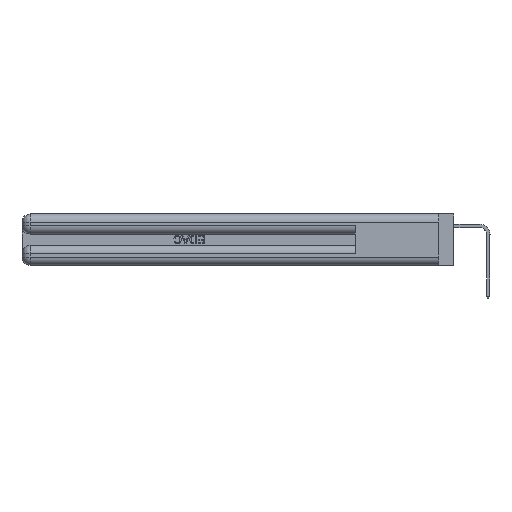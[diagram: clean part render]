
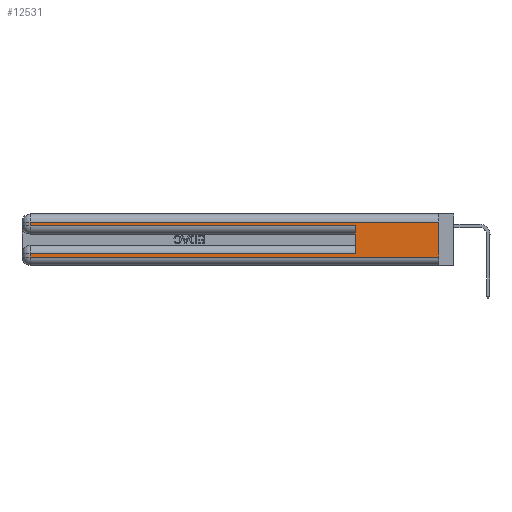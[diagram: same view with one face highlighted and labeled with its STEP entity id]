
A CAD part, left-side view. The second image highlights one B-rep face of the part: STEP entity #12531.
In plain terms, the highlighted planar face has unit normal (-1, 0, 0).
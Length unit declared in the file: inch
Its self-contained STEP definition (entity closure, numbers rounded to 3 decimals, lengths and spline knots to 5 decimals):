
#969 = CARTESIAN_POINT ( 'NONE',  ( 0., 0., 0.06 ) ) ;
#1261 = CARTESIAN_POINT ( 'NONE',  ( 0., 0., 0.37 ) ) ;
#1584 = LINE ( 'NONE', #9420, #37589 ) ;
#1821 = EDGE_CURVE ( 'NONE', #5785, #28528, #43204, .T. ) ;
#3249 = AXIS2_PLACEMENT_3D ( 'NONE', #1261, #8359, #31942 ) ;
#4107 = DIRECTION ( 'NONE',  ( 0., 1., 0. ) ) ;
#5298 = ORIENTED_EDGE ( 'NONE', *, *, #1821, .T. ) ;
#5785 = VERTEX_POINT ( 'NONE', #9802 ) ;
#6307 = VECTOR ( 'NONE', #21690, 39.37008 ) ;
#7692 = VECTOR ( 'NONE', #4107, 39.37008 ) ;
#8278 = EDGE_CURVE ( 'NONE', #22062, #12574, #39935, .T. ) ;
#8359 = DIRECTION ( 'NONE',  ( 1., 0., 0. ) ) ;
#9420 = CARTESIAN_POINT ( 'NONE',  ( 0., 2.94, 0.37 ) ) ;
#9802 = CARTESIAN_POINT ( 'NONE',  ( 0., 2.94, 0.085 ) ) ;
#10342 = CARTESIAN_POINT ( 'NONE',  ( 0., 2.94, 0.37 ) ) ;
#11108 = EDGE_CURVE ( 'NONE', #43314, #23502, #1584, .T. ) ;
#12459 = LINE ( 'NONE', #22307, #20399 ) ;
#12531 = ADVANCED_FACE ( 'NONE', ( #15473 ), #28605, .F. ) ;
#12574 = VERTEX_POINT ( 'NONE', #22025 ) ;
#12840 = DIRECTION ( 'NONE',  ( 0., 0., -1. ) ) ;
#12875 = DIRECTION ( 'NONE',  ( 0., 0., -1. ) ) ;
#13532 = DIRECTION ( 'NONE',  ( 0., -1., 0. ) ) ;
#13911 = CARTESIAN_POINT ( 'NONE',  ( 0., 0.6, 0.085 ) ) ;
#14051 = EDGE_CURVE ( 'NONE', #23502, #34182, #17973, .T. ) ;
#14349 = CARTESIAN_POINT ( 'NONE',  ( 0., 2.94, 0.06 ) ) ;
#15473 = FACE_OUTER_BOUND ( 'NONE', #43568, .T. ) ;
#15482 = CARTESIAN_POINT ( 'NONE',  ( 0., 0., 0.31 ) ) ;
#16345 = VERTEX_POINT ( 'NONE', #13911 ) ;
#16798 = LINE ( 'NONE', #21111, #7692 ) ;
#16910 = VECTOR ( 'NONE', #13532, 39.37008 ) ;
#17183 = DIRECTION ( 'NONE',  ( 0., 0., -1. ) ) ;
#17227 = ORIENTED_EDGE ( 'NONE', *, *, #32364, .T. ) ;
#17973 = LINE ( 'NONE', #20312, #16910 ) ;
#18934 = LINE ( 'NONE', #969, #37772 ) ;
#18978 = CARTESIAN_POINT ( 'NONE',  ( 0., 2.94, 0.31 ) ) ;
#19569 = EDGE_CURVE ( 'NONE', #16345, #5785, #12459, .T. ) ;
#20312 = CARTESIAN_POINT ( 'NONE',  ( 0., 0., 0.285 ) ) ;
#20399 = VECTOR ( 'NONE', #38959, 39.37008 ) ;
#21111 = CARTESIAN_POINT ( 'NONE',  ( 0., 0., 0.31 ) ) ;
#21474 = ORIENTED_EDGE ( 'NONE', *, *, #14051, .T. ) ;
#21554 = CARTESIAN_POINT ( 'NONE',  ( 0., 0.6, 0.145 ) ) ;
#21690 = DIRECTION ( 'NONE',  ( 0., 0., 1. ) ) ;
#22025 = CARTESIAN_POINT ( 'NONE',  ( 0., 0., 0.06 ) ) ;
#22062 = VERTEX_POINT ( 'NONE', #15482 ) ;
#22307 = CARTESIAN_POINT ( 'NONE',  ( 0., 0., 0.085 ) ) ;
#23502 = VERTEX_POINT ( 'NONE', #33559 ) ;
#26377 = CARTESIAN_POINT ( 'NONE',  ( 0., 0., 0.37 ) ) ;
#28528 = VERTEX_POINT ( 'NONE', #14349 ) ;
#28605 = PLANE ( 'NONE',  #3249 ) ;
#30131 = EDGE_CURVE ( 'NONE', #16345, #34182, #33255, .T. ) ;
#31007 = ORIENTED_EDGE ( 'NONE', *, *, #19569, .T. ) ;
#31038 = VECTOR ( 'NONE', #12840, 39.37008 ) ;
#31819 = ORIENTED_EDGE ( 'NONE', *, *, #30131, .F. ) ;
#31942 = DIRECTION ( 'NONE',  ( 0., 0., -1. ) ) ;
#32364 = EDGE_CURVE ( 'NONE', #22062, #43314, #16798, .T. ) ;
#33255 = LINE ( 'NONE', #21554, #6307 ) ;
#33471 = EDGE_CURVE ( 'NONE', #28528, #12574, #18934, .T. ) ;
#33559 = CARTESIAN_POINT ( 'NONE',  ( 0., 2.94, 0.285 ) ) ;
#33992 = ORIENTED_EDGE ( 'NONE', *, *, #33471, .T. ) ;
#34111 = ORIENTED_EDGE ( 'NONE', *, *, #8278, .F. ) ;
#34182 = VERTEX_POINT ( 'NONE', #41712 ) ;
#34297 = VECTOR ( 'NONE', #17183, 39.37008 ) ;
#37589 = VECTOR ( 'NONE', #12875, 39.37008 ) ;
#37772 = VECTOR ( 'NONE', #41482, 39.37008 ) ;
#38959 = DIRECTION ( 'NONE',  ( 0., 1., 0. ) ) ;
#39355 = ORIENTED_EDGE ( 'NONE', *, *, #11108, .T. ) ;
#39935 = LINE ( 'NONE', #26377, #31038 ) ;
#41482 = DIRECTION ( 'NONE',  ( 0., -1., 0. ) ) ;
#41712 = CARTESIAN_POINT ( 'NONE',  ( 0., 0.6, 0.285 ) ) ;
#43204 = LINE ( 'NONE', #10342, #34297 ) ;
#43314 = VERTEX_POINT ( 'NONE', #18978 ) ;
#43568 = EDGE_LOOP ( 'NONE', ( #34111, #17227, #39355, #21474, #31819, #31007, #5298, #33992 ) ) ;
